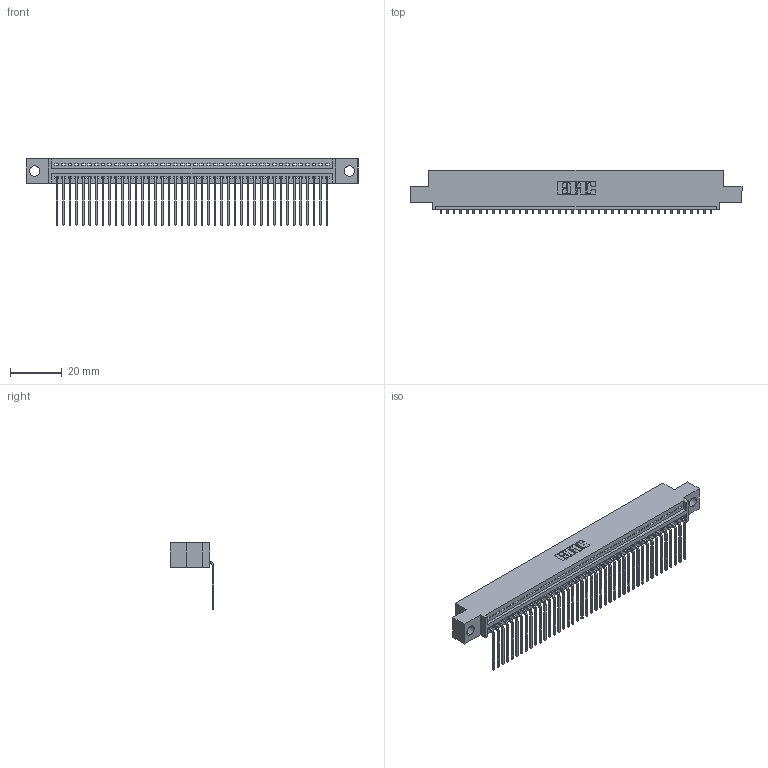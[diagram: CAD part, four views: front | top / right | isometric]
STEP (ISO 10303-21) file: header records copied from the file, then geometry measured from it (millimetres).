
FILE_DESCRIPTION (( 'STEP AP203' ), '1' );
FILE_NAME ('395-042-559-404.STEP', '2021-05-31T15:05:51', ( '' ), ( '' ), 'SwSTEP 2.0', 'SolidWorks 2020', '' );
FILE_SCHEMA (( 'CONFIG_CONTROL_DESIGN' ));
Length unit declared in the file: inch
Products named in the file (3): 395-042-559-404; 345 Part_0.110 Offset - 0.156 Dia-TI; 345-292-001_558 559 Tail - 1
Assembly tree (43 placements, depth 2):
  395-042-559-404
    345 Part_0.110 Offset - 0.156 Dia-TI
    345-292-001_558 559 Tail - 1  x42
Bounding box: 127.89 x 16.75 x 25.53 mm (x, y, z)
Volume: 12107.6 mm3; surface area: 16836.6 mm2
Topology: 43 solids, 43 shells, 2664 faces, 8033 edges, 5298 vertices
Faces by surface type: plane 1862, cylinder 802
Entity records: 32245 total; most frequent: CARTESIAN_POINT 5596, ORIENTED_EDGE 5570, DIRECTION 4885, EDGE_CURVE 2785, LINE 2485, VECTOR 2485, VERTEX_POINT 1854, AXIS2_PLACEMENT_3D 1200
